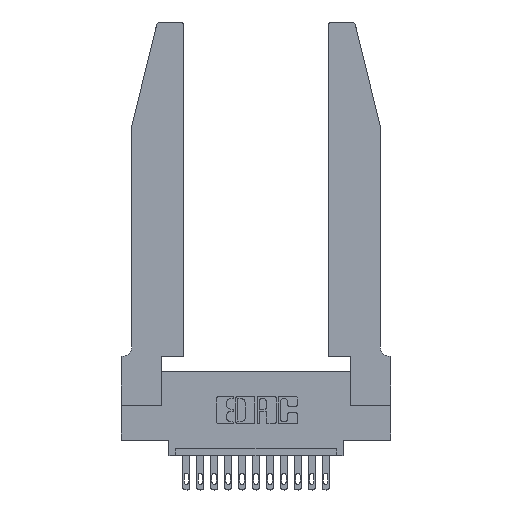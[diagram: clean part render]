
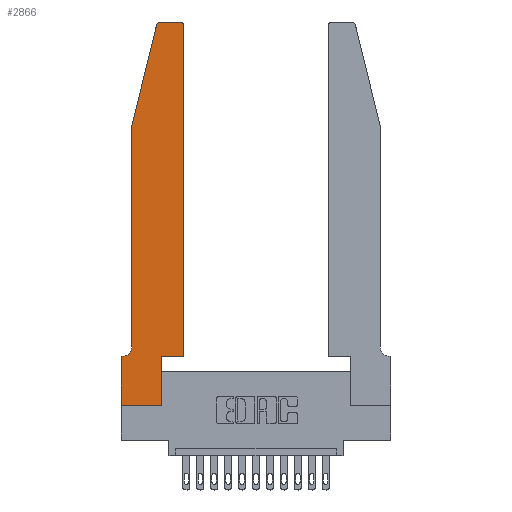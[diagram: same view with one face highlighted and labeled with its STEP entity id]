
A CAD part, top view. The second image highlights one B-rep face of the part: STEP entity #2866.
In plain terms, the highlighted planar face has unit normal (0, 0, 1).
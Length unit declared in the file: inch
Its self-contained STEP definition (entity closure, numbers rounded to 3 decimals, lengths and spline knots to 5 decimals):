
#97 = CARTESIAN_POINT ( 'NONE',  ( 0.25487, 2.72718, 0.37 ) ) ;
#165 = CARTESIAN_POINT ( 'NONE',  ( 0.0755, 0.42, 0.37 ) ) ;
#198 = LINE ( 'NONE', #961, #16477 ) ;
#248 = EDGE_CURVE ( 'NONE', #5505, #8565, #2038, .T. ) ;
#590 = VERTEX_POINT ( 'NONE', #97 ) ;
#697 = FACE_OUTER_BOUND ( 'NONE', #3142, .T. ) ;
#961 = CARTESIAN_POINT ( 'NONE',  ( 0.0755, 2., 0.37 ) ) ;
#1247 = CIRCLE ( 'NONE', #11471, 0.03 ) ;
#1279 = VECTOR ( 'NONE', #4923, 39.37008 ) ;
#1317 = DIRECTION ( 'NONE',  ( 0., 0., 1. ) ) ;
#1380 = DIRECTION ( 'NONE',  ( 1., 0., 0. ) ) ;
#1408 = VECTOR ( 'NONE', #1599, 39.37008 ) ;
#1476 = DIRECTION ( 'NONE',  ( 0., -1., 0. ) ) ;
#1514 = CARTESIAN_POINT ( 'NONE',  ( 0.4505, 0.35, 0.37 ) ) ;
#1599 = DIRECTION ( 'NONE',  ( -1., 0., 0. ) ) ;
#2038 = LINE ( 'NONE', #3524, #15129 ) ;
#2085 = EDGE_CURVE ( 'NONE', #8565, #3976, #14083, .T. ) ;
#2675 = CARTESIAN_POINT ( 'NONE',  ( 0.0755, 0.35, 0.37 ) ) ;
#2866 = ADVANCED_FACE ( 'NONE', ( #697 ), #9211, .T. ) ;
#3036 = CARTESIAN_POINT ( 'NONE',  ( 0.0055, 0.42, 0.37 ) ) ;
#3142 = EDGE_LOOP ( 'NONE', ( #9098, #13262, #14400, #13108, #9405, #3276, #13032, #11926, #7760, #8566, #16131, #15935 ) ) ;
#3276 = ORIENTED_EDGE ( 'NONE', *, *, #11549, .T. ) ;
#3524 = CARTESIAN_POINT ( 'NONE',  ( 0.2865, 0.35, 0.37 ) ) ;
#3541 = LINE ( 'NONE', #2675, #11031 ) ;
#3696 = CARTESIAN_POINT ( 'NONE',  ( 0.4205, 2.75, 0.37 ) ) ;
#3976 = VERTEX_POINT ( 'NONE', #15969 ) ;
#4045 = CARTESIAN_POINT ( 'NONE',  ( 0., 0., 0.37 ) ) ;
#4103 = VECTOR ( 'NONE', #1476, 39.37008 ) ;
#4160 = DIRECTION ( 'NONE',  ( 1., 0., 0. ) ) ;
#4389 = DIRECTION ( 'NONE',  ( -1., 0., 0. ) ) ;
#4489 = CARTESIAN_POINT ( 'NONE',  ( 0., 0., 0.37 ) ) ;
#4685 = CARTESIAN_POINT ( 'NONE',  ( 0., 0., 0.37 ) ) ;
#4788 = DIRECTION ( 'NONE',  ( 0., 0., 1. ) ) ;
#4816 = VERTEX_POINT ( 'NONE', #15954 ) ;
#4905 = CARTESIAN_POINT ( 'NONE',  ( 0.2865, 0.35, 0.37 ) ) ;
#4923 = DIRECTION ( 'NONE',  ( 0., -1., 0. ) ) ;
#4928 = AXIS2_PLACEMENT_3D ( 'NONE', #9916, #4788, #16505 ) ;
#5126 = CARTESIAN_POINT ( 'NONE',  ( 0.4505, 0.35, 0.37 ) ) ;
#5505 = VERTEX_POINT ( 'NONE', #7582 ) ;
#5683 = CARTESIAN_POINT ( 'NONE',  ( 0.2605, 2.75, 0.37 ) ) ;
#5792 = VECTOR ( 'NONE', #11773, 39.37008 ) ;
#6301 = CARTESIAN_POINT ( 'NONE',  ( 0.4505, 2.72, 0.37 ) ) ;
#6364 = CARTESIAN_POINT ( 'NONE',  ( 0.284, 2.72, 0.37 ) ) ;
#6766 = VECTOR ( 'NONE', #4160, 39.37008 ) ;
#6825 = LINE ( 'NONE', #1514, #16998 ) ;
#7370 = CARTESIAN_POINT ( 'NONE',  ( 0., 0.35, 0.37 ) ) ;
#7582 = CARTESIAN_POINT ( 'NONE',  ( 0.2865, 0., 0.37 ) ) ;
#7584 = VERTEX_POINT ( 'NONE', #165 ) ;
#7587 = CARTESIAN_POINT ( 'NONE',  ( 0.0755, 2., 0.37 ) ) ;
#7667 = LINE ( 'NONE', #13385, #4103 ) ;
#7684 = DIRECTION ( 'NONE',  ( 1., 0., 0. ) ) ;
#7760 = ORIENTED_EDGE ( 'NONE', *, *, #248, .T. ) ;
#8026 = VERTEX_POINT ( 'NONE', #7370 ) ;
#8261 = DIRECTION ( 'NONE',  ( 0., 1., 0. ) ) ;
#8565 = VERTEX_POINT ( 'NONE', #4905 ) ;
#8566 = ORIENTED_EDGE ( 'NONE', *, *, #2085, .T. ) ;
#8727 = LINE ( 'NONE', #5683, #1408 ) ;
#9050 = DIRECTION ( 'NONE',  ( 0., 0., 1. ) ) ;
#9080 = AXIS2_PLACEMENT_3D ( 'NONE', #11846, #1317, #1380 ) ;
#9098 = ORIENTED_EDGE ( 'NONE', *, *, #13803, .T. ) ;
#9135 = DIRECTION ( 'NONE',  ( -0.239, -0.971, 0. ) ) ;
#9211 = PLANE ( 'NONE',  #9080 ) ;
#9405 = ORIENTED_EDGE ( 'NONE', *, *, #13179, .T. ) ;
#9409 = LINE ( 'NONE', #4045, #6766 ) ;
#9916 = CARTESIAN_POINT ( 'NONE',  ( 0.4205, 2.72, 0.37 ) ) ;
#10130 = EDGE_CURVE ( 'NONE', #8026, #12465, #15455, .T. ) ;
#10285 = EDGE_CURVE ( 'NONE', #14724, #14207, #11517, .T. ) ;
#10407 = VERTEX_POINT ( 'NONE', #16785 ) ;
#10430 = EDGE_CURVE ( 'NONE', #12465, #5505, #9409, .T. ) ;
#11031 = VECTOR ( 'NONE', #11944, 39.37008 ) ;
#11052 = EDGE_CURVE ( 'NONE', #4816, #590, #1247, .T. ) ;
#11316 = VERTEX_POINT ( 'NONE', #7587 ) ;
#11471 = AXIS2_PLACEMENT_3D ( 'NONE', #6364, #9050, #7684 ) ;
#11517 = CIRCLE ( 'NONE', #4928, 0.03 ) ;
#11549 = EDGE_CURVE ( 'NONE', #10407, #8026, #3541, .T. ) ;
#11773 = DIRECTION ( 'NONE',  ( 1., 0., 0. ) ) ;
#11846 = CARTESIAN_POINT ( 'NONE',  ( 0., 0.35, 0.37 ) ) ;
#11926 = ORIENTED_EDGE ( 'NONE', *, *, #10430, .T. ) ;
#11944 = DIRECTION ( 'NONE',  ( -1., 0., 0. ) ) ;
#12036 = EDGE_CURVE ( 'NONE', #590, #11316, #198, .T. ) ;
#12307 = CIRCLE ( 'NONE', #13272, 0.07 ) ;
#12364 = DIRECTION ( 'NONE',  ( 0., 0., -1. ) ) ;
#12465 = VERTEX_POINT ( 'NONE', #4489 ) ;
#13032 = ORIENTED_EDGE ( 'NONE', *, *, #10130, .T. ) ;
#13108 = ORIENTED_EDGE ( 'NONE', *, *, #15546, .T. ) ;
#13179 = EDGE_CURVE ( 'NONE', #7584, #10407, #12307, .T. ) ;
#13262 = ORIENTED_EDGE ( 'NONE', *, *, #11052, .T. ) ;
#13272 = AXIS2_PLACEMENT_3D ( 'NONE', #3036, #12364, #4389 ) ;
#13385 = CARTESIAN_POINT ( 'NONE',  ( 0.0755, 2., 0.37 ) ) ;
#13803 = EDGE_CURVE ( 'NONE', #14207, #4816, #8727, .T. ) ;
#14083 = LINE ( 'NONE', #5126, #5792 ) ;
#14190 = DIRECTION ( 'NONE',  ( 0., 1., 0. ) ) ;
#14207 = VERTEX_POINT ( 'NONE', #3696 ) ;
#14400 = ORIENTED_EDGE ( 'NONE', *, *, #12036, .T. ) ;
#14724 = VERTEX_POINT ( 'NONE', #6301 ) ;
#15129 = VECTOR ( 'NONE', #14190, 39.37008 ) ;
#15455 = LINE ( 'NONE', #4685, #1279 ) ;
#15546 = EDGE_CURVE ( 'NONE', #11316, #7584, #7667, .T. ) ;
#15935 = ORIENTED_EDGE ( 'NONE', *, *, #10285, .T. ) ;
#15954 = CARTESIAN_POINT ( 'NONE',  ( 0.284, 2.75, 0.37 ) ) ;
#15969 = CARTESIAN_POINT ( 'NONE',  ( 0.4505, 0.35, 0.37 ) ) ;
#16131 = ORIENTED_EDGE ( 'NONE', *, *, #16188, .T. ) ;
#16188 = EDGE_CURVE ( 'NONE', #3976, #14724, #6825, .T. ) ;
#16477 = VECTOR ( 'NONE', #9135, 39.37008 ) ;
#16505 = DIRECTION ( 'NONE',  ( 1., 0., 0. ) ) ;
#16785 = CARTESIAN_POINT ( 'NONE',  ( 0.0055, 0.35, 0.37 ) ) ;
#16998 = VECTOR ( 'NONE', #8261, 39.37008 ) ;
